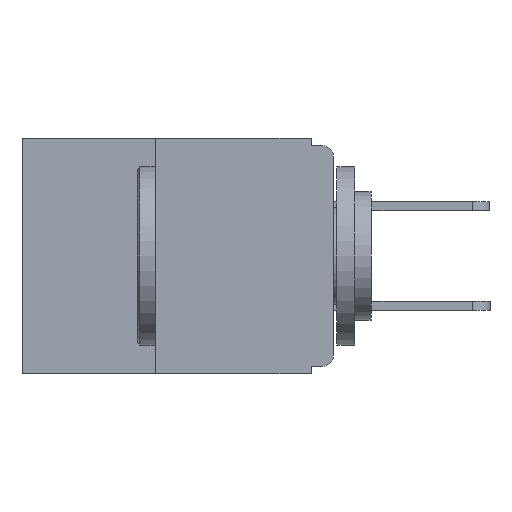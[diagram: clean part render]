
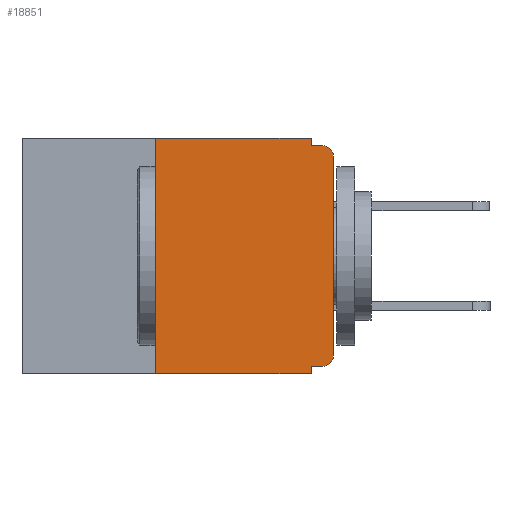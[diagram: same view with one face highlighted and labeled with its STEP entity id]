
A CAD part, left-side view. The second image highlights one B-rep face of the part: STEP entity #18851.
In plain terms, the highlighted planar face has unit normal (-1, 0, 0).
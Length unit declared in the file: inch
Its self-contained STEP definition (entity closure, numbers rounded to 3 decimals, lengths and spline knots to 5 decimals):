
#280 = VERTEX_POINT ( 'NONE', #4640 ) ;
#338 = CARTESIAN_POINT ( 'NONE',  ( 0., 0., 0. ) ) ;
#817 = DIRECTION ( 'NONE',  ( 0., 0., -1. ) ) ;
#1527 = DIRECTION ( 'NONE',  ( 0., 0., -1. ) ) ;
#2363 = ORIENTED_EDGE ( 'NONE', *, *, #19548, .T. ) ;
#2562 = CARTESIAN_POINT ( 'NONE',  ( 0., 0., -0.32 ) ) ;
#2766 = LINE ( 'NONE', #2782, #27812 ) ;
#2782 = CARTESIAN_POINT ( 'NONE',  ( 0., 0.437, 0. ) ) ;
#2867 = DIRECTION ( 'NONE',  ( 0., 0., 1. ) ) ;
#3776 = VECTOR ( 'NONE', #18073, 39.37008 ) ;
#4640 = CARTESIAN_POINT ( 'NONE',  ( 0., 0.031, 0. ) ) ;
#4737 = AXIS2_PLACEMENT_3D ( 'NONE', #30531, #16352, #1527 ) ;
#4856 = CARTESIAN_POINT ( 'NONE',  ( 0., 0.25, -0.33 ) ) ;
#5147 = DIRECTION ( 'NONE',  ( 0., 1., 0. ) ) ;
#5282 = VECTOR ( 'NONE', #27435, 39.37008 ) ;
#5353 = DIRECTION ( 'NONE',  ( 0., -1., 0. ) ) ;
#5588 = ORIENTED_EDGE ( 'NONE', *, *, #9992, .F. ) ;
#5981 = CARTESIAN_POINT ( 'NONE',  ( 0., 0.031, 0. ) ) ;
#6582 = CARTESIAN_POINT ( 'NONE',  ( 0., 0.031, -0.33 ) ) ;
#7009 = ORIENTED_EDGE ( 'NONE', *, *, #17866, .F. ) ;
#7373 = DIRECTION ( 'NONE',  ( 0., 0., 1. ) ) ;
#7615 = LINE ( 'NONE', #20388, #5282 ) ;
#8535 = DIRECTION ( 'NONE',  ( -1., 0., 0. ) ) ;
#8810 = CARTESIAN_POINT ( 'NONE',  ( 0., 0.015, -0.32 ) ) ;
#9719 = LINE ( 'NONE', #338, #28037 ) ;
#9992 = EDGE_CURVE ( 'NONE', #12372, #27329, #29445, .T. ) ;
#10606 = CARTESIAN_POINT ( 'NONE',  ( 0., 0.25, 0. ) ) ;
#10903 = AXIS2_PLACEMENT_3D ( 'NONE', #23027, #8535, #25379 ) ;
#11002 = LINE ( 'NONE', #2562, #16625 ) ;
#11543 = FACE_OUTER_BOUND ( 'NONE', #26776, .T. ) ;
#12372 = VERTEX_POINT ( 'NONE', #21990 ) ;
#13479 = VECTOR ( 'NONE', #7373, 39.37008 ) ;
#13507 = VERTEX_POINT ( 'NONE', #6582 ) ;
#13779 = EDGE_CURVE ( 'NONE', #22353, #280, #2766, .T. ) ;
#13808 = CARTESIAN_POINT ( 'NONE',  ( 0., 0.031, -0.32 ) ) ;
#14081 = CARTESIAN_POINT ( 'NONE',  ( 0., 0.25, -0.33 ) ) ;
#14443 = VECTOR ( 'NONE', #20716, 39.37008 ) ;
#14879 = DIRECTION ( 'NONE',  ( 1., 0., 0. ) ) ;
#15469 = EDGE_CURVE ( 'NONE', #27478, #17936, #30288, .T. ) ;
#15772 = ORIENTED_EDGE ( 'NONE', *, *, #26663, .F. ) ;
#16352 = DIRECTION ( 'NONE',  ( -1., 0., 0. ) ) ;
#16598 = AXIS2_PLACEMENT_3D ( 'NONE', #24405, #14879, #31407 ) ;
#16625 = VECTOR ( 'NONE', #5147, 39.37008 ) ;
#17866 = EDGE_CURVE ( 'NONE', #21400, #13507, #25784, .T. ) ;
#17936 = VERTEX_POINT ( 'NONE', #25801 ) ;
#18073 = DIRECTION ( 'NONE',  ( 0., -1., 0. ) ) ;
#18851 = ADVANCED_FACE ( 'NONE', ( #11543 ), #26672, .F. ) ;
#19338 = VERTEX_POINT ( 'NONE', #23765 ) ;
#19519 = VECTOR ( 'NONE', #817, 39.37008 ) ;
#19548 = EDGE_CURVE ( 'NONE', #19805, #13507, #7615, .T. ) ;
#19805 = VERTEX_POINT ( 'NONE', #14081 ) ;
#19817 = ORIENTED_EDGE ( 'NONE', *, *, #13779, .F. ) ;
#19847 = ORIENTED_EDGE ( 'NONE', *, *, #22944, .T. ) ;
#20382 = EDGE_CURVE ( 'NONE', #19338, #27329, #26780, .T. ) ;
#20388 = CARTESIAN_POINT ( 'NONE',  ( 0., 0.437, -0.33 ) ) ;
#20546 = CARTESIAN_POINT ( 'NONE',  ( 0., 0., -0.01 ) ) ;
#20716 = DIRECTION ( 'NONE',  ( 0., 0., -1. ) ) ;
#21385 = ORIENTED_EDGE ( 'NONE', *, *, #24283, .F. ) ;
#21400 = VERTEX_POINT ( 'NONE', #13808 ) ;
#21645 = LINE ( 'NONE', #5981, #14443 ) ;
#21990 = CARTESIAN_POINT ( 'NONE',  ( 0., 0.031, -0.01 ) ) ;
#22353 = VERTEX_POINT ( 'NONE', #10606 ) ;
#22944 = EDGE_CURVE ( 'NONE', #17936, #19338, #9719, .T. ) ;
#23027 = CARTESIAN_POINT ( 'NONE',  ( 0., 0.015, -0.305 ) ) ;
#23765 = CARTESIAN_POINT ( 'NONE',  ( 0., 0., -0.025 ) ) ;
#24283 = EDGE_CURVE ( 'NONE', #19805, #22353, #26200, .T. ) ;
#24405 = CARTESIAN_POINT ( 'NONE',  ( 0., 0.437, 0. ) ) ;
#25018 = CARTESIAN_POINT ( 'NONE',  ( 0., 0.015, -0.01 ) ) ;
#25379 = DIRECTION ( 'NONE',  ( 0., 0., -1. ) ) ;
#25784 = LINE ( 'NONE', #29922, #19519 ) ;
#25801 = CARTESIAN_POINT ( 'NONE',  ( 0., 0., -0.305 ) ) ;
#25861 = EDGE_CURVE ( 'NONE', #280, #12372, #21645, .T. ) ;
#26092 = ORIENTED_EDGE ( 'NONE', *, *, #15469, .T. ) ;
#26200 = LINE ( 'NONE', #4856, #13479 ) ;
#26663 = EDGE_CURVE ( 'NONE', #27478, #21400, #11002, .T. ) ;
#26672 = PLANE ( 'NONE',  #16598 ) ;
#26776 = EDGE_LOOP ( 'NONE', ( #19847, #30316, #5588, #29428, #19817, #21385, #2363, #7009, #15772, #26092 ) ) ;
#26780 = CIRCLE ( 'NONE', #4737, 0.015 ) ;
#27329 = VERTEX_POINT ( 'NONE', #25018 ) ;
#27435 = DIRECTION ( 'NONE',  ( 0., -1., 0. ) ) ;
#27478 = VERTEX_POINT ( 'NONE', #8810 ) ;
#27812 = VECTOR ( 'NONE', #5353, 39.37008 ) ;
#28037 = VECTOR ( 'NONE', #2867, 39.37008 ) ;
#29428 = ORIENTED_EDGE ( 'NONE', *, *, #25861, .F. ) ;
#29445 = LINE ( 'NONE', #20546, #3776 ) ;
#29922 = CARTESIAN_POINT ( 'NONE',  ( 0., 0.031, -0.33 ) ) ;
#30288 = CIRCLE ( 'NONE', #10903, 0.015 ) ;
#30316 = ORIENTED_EDGE ( 'NONE', *, *, #20382, .T. ) ;
#30531 = CARTESIAN_POINT ( 'NONE',  ( 0., 0.015, -0.025 ) ) ;
#31407 = DIRECTION ( 'NONE',  ( 0., 0., -1. ) ) ;
